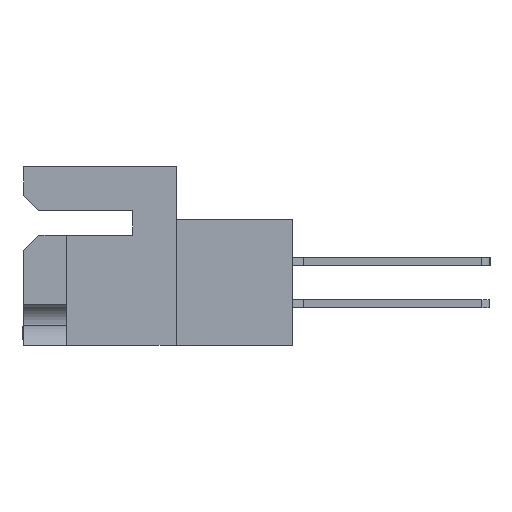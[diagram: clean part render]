
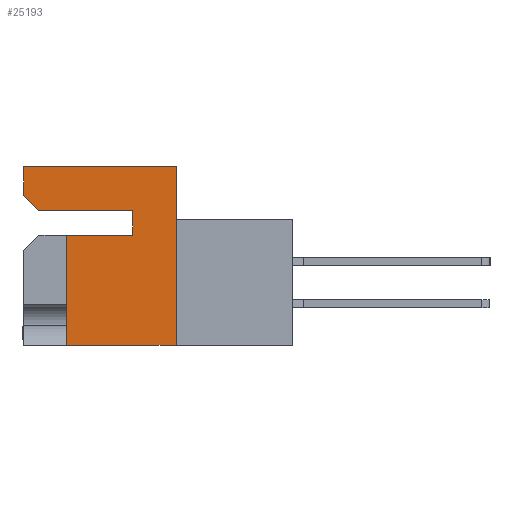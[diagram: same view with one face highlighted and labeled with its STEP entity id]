
A CAD part, left-side view. The second image highlights one B-rep face of the part: STEP entity #25193.
In plain terms, the highlighted planar face has unit normal (-1, 0, 0).
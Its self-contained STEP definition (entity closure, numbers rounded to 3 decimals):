
#1339 = PLANE ( 'NONE',  #21049 ) ;
#1400 = VECTOR ( 'NONE', #10619, 1000. ) ;
#1442 = CARTESIAN_POINT ( 'NONE',  ( 0., 0., -3.302 ) ) ;
#1560 = DIRECTION ( 'NONE',  ( 0., 1., 0. ) ) ;
#1946 = CARTESIAN_POINT ( 'NONE',  ( 0., 11.506, 0. ) ) ;
#2102 = CARTESIAN_POINT ( 'NONE',  ( 0., 8.255, -13.487 ) ) ;
#3917 = EDGE_CURVE ( 'NONE', #9250, #20340, #13041, .T. ) ;
#4384 = CARTESIAN_POINT ( 'NONE',  ( 0., 8.255, -5.182 ) ) ;
#4543 = EDGE_CURVE ( 'NONE', #11981, #23313, #35088, .T. ) ;
#4707 = CARTESIAN_POINT ( 'NONE',  ( 0., 3.251, -5.182 ) ) ;
#4852 = ORIENTED_EDGE ( 'NONE', *, *, #15066, .F. ) ;
#5323 = LINE ( 'NONE', #34358, #21509 ) ;
#5900 = EDGE_LOOP ( 'NONE', ( #17121, #20972, #13425, #20890, #16220, #34301, #24374, #4852, #14927 ) ) ;
#6567 = CARTESIAN_POINT ( 'NONE',  ( 0., 11.506, -13.487 ) ) ;
#7139 = CARTESIAN_POINT ( 'NONE',  ( 0., 11.506, 0. ) ) ;
#7383 = LINE ( 'NONE', #29519, #1400 ) ;
#7495 = DIRECTION ( 'NONE',  ( 0., 0., -1. ) ) ;
#8348 = CARTESIAN_POINT ( 'NONE',  ( 0., 3.251, -5.182 ) ) ;
#8519 = CARTESIAN_POINT ( 'NONE',  ( 0., 10.363, -3.302 ) ) ;
#9250 = VERTEX_POINT ( 'NONE', #7139 ) ;
#10291 = EDGE_CURVE ( 'NONE', #20340, #14775, #5323, .T. ) ;
#10547 = LINE ( 'NONE', #21880, #22456 ) ;
#10619 = DIRECTION ( 'NONE',  ( 0., 0., 1. ) ) ;
#11037 = VECTOR ( 'NONE', #27521, 1000. ) ;
#11576 = CARTESIAN_POINT ( 'NONE',  ( 0., 3.251, -3.302 ) ) ;
#11826 = DIRECTION ( 'NONE',  ( 0., 0., 1. ) ) ;
#11981 = VERTEX_POINT ( 'NONE', #4707 ) ;
#12061 = VERTEX_POINT ( 'NONE', #2102 ) ;
#12186 = CARTESIAN_POINT ( 'NONE',  ( 0., 0., 0. ) ) ;
#12638 = DIRECTION ( 'NONE',  ( 1., 0., 0. ) ) ;
#13041 = LINE ( 'NONE', #1946, #29610 ) ;
#13113 = DIRECTION ( 'NONE',  ( 0., 0., -1. ) ) ;
#13425 = ORIENTED_EDGE ( 'NONE', *, *, #3917, .F. ) ;
#14260 = VECTOR ( 'NONE', #24971, 1000. ) ;
#14775 = VERTEX_POINT ( 'NONE', #22097 ) ;
#14927 = ORIENTED_EDGE ( 'NONE', *, *, #27543, .F. ) ;
#15066 = EDGE_CURVE ( 'NONE', #28922, #11981, #29707, .T. ) ;
#16220 = ORIENTED_EDGE ( 'NONE', *, *, #23315, .T. ) ;
#17121 = ORIENTED_EDGE ( 'NONE', *, *, #23913, .F. ) ;
#18884 = DIRECTION ( 'NONE',  ( 0., 1., 0. ) ) ;
#19093 = LINE ( 'NONE', #8519, #11037 ) ;
#19797 = VECTOR ( 'NONE', #11826, 1000. ) ;
#19901 = VECTOR ( 'NONE', #21216, 1000. ) ;
#20340 = VERTEX_POINT ( 'NONE', #27198 ) ;
#20890 = ORIENTED_EDGE ( 'NONE', *, *, #30514, .F. ) ;
#20972 = ORIENTED_EDGE ( 'NONE', *, *, #10291, .F. ) ;
#21049 = AXIS2_PLACEMENT_3D ( 'NONE', #12186, #12638, #13113 ) ;
#21216 = DIRECTION ( 'NONE',  ( 0., -1., 0. ) ) ;
#21509 = VECTOR ( 'NONE', #7495, 1000. ) ;
#21880 = CARTESIAN_POINT ( 'NONE',  ( 0., -8.814, -13.487 ) ) ;
#22097 = CARTESIAN_POINT ( 'NONE',  ( 0., 0., -13.487 ) ) ;
#22456 = VECTOR ( 'NONE', #18884, 1000. ) ;
#23263 = CARTESIAN_POINT ( 'NONE',  ( 0., 0., -5.182 ) ) ;
#23313 = VERTEX_POINT ( 'NONE', #11576 ) ;
#23315 = EDGE_CURVE ( 'NONE', #26110, #34130, #19093, .T. ) ;
#23366 = DIRECTION ( 'NONE',  ( 0., -1., 0. ) ) ;
#23913 = EDGE_CURVE ( 'NONE', #14775, #12061, #10547, .T. ) ;
#24374 = ORIENTED_EDGE ( 'NONE', *, *, #4543, .F. ) ;
#24706 = VECTOR ( 'NONE', #1560, 1000. ) ;
#24971 = DIRECTION ( 'NONE',  ( 0., 0., 1. ) ) ;
#25193 = ADVANCED_FACE ( 'NONE', ( #27988 ), #1339, .F. ) ;
#26110 = VERTEX_POINT ( 'NONE', #31739 ) ;
#26174 = LINE ( 'NONE', #6567, #19797 ) ;
#27198 = CARTESIAN_POINT ( 'NONE',  ( 0., 0., 0. ) ) ;
#27521 = DIRECTION ( 'NONE',  ( 0., -0.707, -0.707 ) ) ;
#27543 = EDGE_CURVE ( 'NONE', #12061, #28922, #7383, .T. ) ;
#27988 = FACE_OUTER_BOUND ( 'NONE', #5900, .T. ) ;
#28922 = VERTEX_POINT ( 'NONE', #4384 ) ;
#29519 = CARTESIAN_POINT ( 'NONE',  ( 0., 8.255, -5.182 ) ) ;
#29610 = VECTOR ( 'NONE', #23366, 1000. ) ;
#29707 = LINE ( 'NONE', #23263, #19901 ) ;
#30514 = EDGE_CURVE ( 'NONE', #26110, #9250, #26174, .T. ) ;
#31739 = CARTESIAN_POINT ( 'NONE',  ( 0., 11.506, -2.159 ) ) ;
#32193 = CARTESIAN_POINT ( 'NONE',  ( 0., 10.363, -3.302 ) ) ;
#33484 = EDGE_CURVE ( 'NONE', #23313, #34130, #34479, .T. ) ;
#34130 = VERTEX_POINT ( 'NONE', #32193 ) ;
#34301 = ORIENTED_EDGE ( 'NONE', *, *, #33484, .F. ) ;
#34358 = CARTESIAN_POINT ( 'NONE',  ( 0., 0., 0. ) ) ;
#34479 = LINE ( 'NONE', #1442, #24706 ) ;
#35088 = LINE ( 'NONE', #8348, #14260 ) ;
